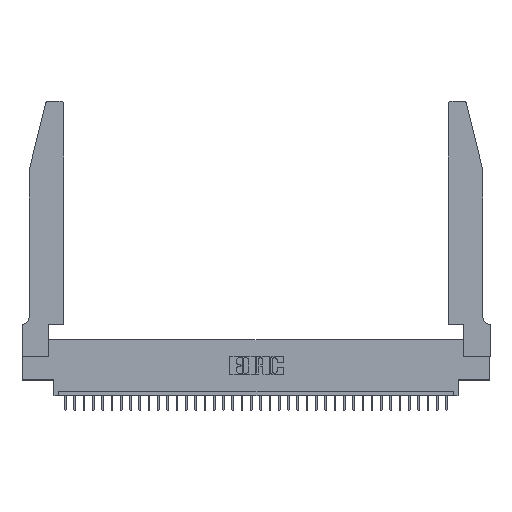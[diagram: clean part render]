
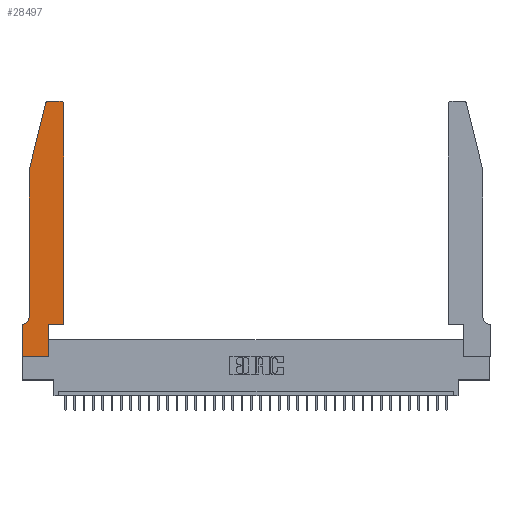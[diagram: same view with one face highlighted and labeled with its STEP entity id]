
A CAD part, top view. The second image highlights one B-rep face of the part: STEP entity #28497.
In plain terms, the highlighted planar face has unit normal (0, 0, 1).
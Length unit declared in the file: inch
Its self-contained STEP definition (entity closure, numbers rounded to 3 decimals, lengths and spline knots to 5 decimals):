
#23 = AXIS2_PLACEMENT_3D ( 'NONE', #22411, #19814, #30839 ) ;
#303 = DIRECTION ( 'NONE',  ( 0., 0., 1. ) ) ;
#573 = LINE ( 'NONE', #972, #12017 ) ;
#666 = EDGE_CURVE ( 'NONE', #1875, #23000, #20949, .T. ) ;
#972 = CARTESIAN_POINT ( 'NONE',  ( 0.2865, 0.35, 0.37 ) ) ;
#1875 = VERTEX_POINT ( 'NONE', #16837 ) ;
#1947 = PLANE ( 'NONE',  #32870 ) ;
#2014 = CARTESIAN_POINT ( 'NONE',  ( 0.4505, 0.35, 0.37 ) ) ;
#2196 = DIRECTION ( 'NONE',  ( 0., 1., 0. ) ) ;
#2394 = CARTESIAN_POINT ( 'NONE',  ( 0.4505, 2.72, 0.37 ) ) ;
#2555 = LINE ( 'NONE', #10203, #13099 ) ;
#2617 = CARTESIAN_POINT ( 'NONE',  ( 0.4205, 2.72, 0.37 ) ) ;
#2814 = EDGE_CURVE ( 'NONE', #3935, #32308, #13281, .T. ) ;
#2933 = EDGE_CURVE ( 'NONE', #7395, #24119, #9731, .T. ) ;
#3104 = CARTESIAN_POINT ( 'NONE',  ( 0., 0.35, 0.37 ) ) ;
#3274 = DIRECTION ( 'NONE',  ( 0., 0., 1. ) ) ;
#3289 = VERTEX_POINT ( 'NONE', #25113 ) ;
#3935 = VERTEX_POINT ( 'NONE', #27702 ) ;
#4242 = DIRECTION ( 'NONE',  ( -0.239, -0.971, 0. ) ) ;
#4882 = EDGE_CURVE ( 'NONE', #5404, #3289, #2555, .T. ) ;
#5018 = CARTESIAN_POINT ( 'NONE',  ( 0.0055, 0.35, 0.37 ) ) ;
#5260 = CIRCLE ( 'NONE', #9674, 0.03 ) ;
#5404 = VERTEX_POINT ( 'NONE', #26618 ) ;
#5456 = LINE ( 'NONE', #9632, #30645 ) ;
#6703 = VERTEX_POINT ( 'NONE', #7307 ) ;
#7047 = EDGE_CURVE ( 'NONE', #10008, #7395, #35138, .T. ) ;
#7307 = CARTESIAN_POINT ( 'NONE',  ( 0.2865, 0., 0.37 ) ) ;
#7395 = VERTEX_POINT ( 'NONE', #3104 ) ;
#7493 = EDGE_CURVE ( 'NONE', #24119, #6703, #25794, .T. ) ;
#7715 = VECTOR ( 'NONE', #22117, 39.37008 ) ;
#7849 = DIRECTION ( 'NONE',  ( 1., 0., 0. ) ) ;
#8033 = EDGE_CURVE ( 'NONE', #6703, #1875, #573, .T. ) ;
#9632 = CARTESIAN_POINT ( 'NONE',  ( 0.0755, 2., 0.37 ) ) ;
#9674 = AXIS2_PLACEMENT_3D ( 'NONE', #2617, #3274, #16997 ) ;
#9731 = LINE ( 'NONE', #20816, #12389 ) ;
#10008 = VERTEX_POINT ( 'NONE', #5018 ) ;
#10203 = CARTESIAN_POINT ( 'NONE',  ( 0.0755, 2., 0.37 ) ) ;
#10679 = CARTESIAN_POINT ( 'NONE',  ( 0., 0.35, 0.37 ) ) ;
#11181 = ORIENTED_EDGE ( 'NONE', *, *, #14940, .T. ) ;
#11901 = CARTESIAN_POINT ( 'NONE',  ( 0.2605, 2.75, 0.37 ) ) ;
#12017 = VECTOR ( 'NONE', #2196, 39.37008 ) ;
#12389 = VECTOR ( 'NONE', #12514, 39.37008 ) ;
#12490 = DIRECTION ( 'NONE',  ( -1., 0., 0. ) ) ;
#12514 = DIRECTION ( 'NONE',  ( 0., -1., 0. ) ) ;
#12538 = CARTESIAN_POINT ( 'NONE',  ( 0.284, 2.75, 0.37 ) ) ;
#13099 = VECTOR ( 'NONE', #26910, 39.37008 ) ;
#13281 = LINE ( 'NONE', #11901, #23899 ) ;
#13383 = DIRECTION ( 'NONE',  ( 1., 0., 0. ) ) ;
#13661 = VERTEX_POINT ( 'NONE', #25826 ) ;
#14126 = ORIENTED_EDGE ( 'NONE', *, *, #2814, .T. ) ;
#14582 = ORIENTED_EDGE ( 'NONE', *, *, #21919, .T. ) ;
#14605 = VECTOR ( 'NONE', #19224, 39.37008 ) ;
#14940 = EDGE_CURVE ( 'NONE', #23000, #23074, #34547, .T. ) ;
#15252 = ORIENTED_EDGE ( 'NONE', *, *, #666, .T. ) ;
#16066 = VECTOR ( 'NONE', #24854, 39.37008 ) ;
#16837 = CARTESIAN_POINT ( 'NONE',  ( 0.2865, 0.35, 0.37 ) ) ;
#16997 = DIRECTION ( 'NONE',  ( 1., 0., 0. ) ) ;
#17340 = ORIENTED_EDGE ( 'NONE', *, *, #8033, .T. ) ;
#17452 = CARTESIAN_POINT ( 'NONE',  ( 0.0755, 0.35, 0.37 ) ) ;
#18187 = ORIENTED_EDGE ( 'NONE', *, *, #30201, .T. ) ;
#19224 = DIRECTION ( 'NONE',  ( 0., 1., 0. ) ) ;
#19736 = EDGE_CURVE ( 'NONE', #32308, #13661, #23760, .T. ) ;
#19814 = DIRECTION ( 'NONE',  ( 0., 0., -1. ) ) ;
#20065 = VECTOR ( 'NONE', #12490, 39.37008 ) ;
#20454 = DIRECTION ( 'NONE',  ( -1., 0., 0. ) ) ;
#20494 = ORIENTED_EDGE ( 'NONE', *, *, #7493, .T. ) ;
#20816 = CARTESIAN_POINT ( 'NONE',  ( 0., 0., 0.37 ) ) ;
#20949 = LINE ( 'NONE', #26591, #7715 ) ;
#21100 = ORIENTED_EDGE ( 'NONE', *, *, #7047, .T. ) ;
#21771 = EDGE_LOOP ( 'NONE', ( #14126, #31903, #14582, #31843, #32867, #21100, #32551, #20494, #17340, #15252, #11181, #18187 ) ) ;
#21919 = EDGE_CURVE ( 'NONE', #13661, #5404, #5456, .T. ) ;
#22117 = DIRECTION ( 'NONE',  ( 1., 0., 0. ) ) ;
#22411 = CARTESIAN_POINT ( 'NONE',  ( 0.0055, 0.42, 0.37 ) ) ;
#23000 = VERTEX_POINT ( 'NONE', #2014 ) ;
#23049 = FACE_OUTER_BOUND ( 'NONE', #21771, .T. ) ;
#23074 = VERTEX_POINT ( 'NONE', #2394 ) ;
#23760 = CIRCLE ( 'NONE', #34315, 0.03 ) ;
#23899 = VECTOR ( 'NONE', #20454, 39.37008 ) ;
#24119 = VERTEX_POINT ( 'NONE', #29345 ) ;
#24854 = DIRECTION ( 'NONE',  ( 1., 0., 0. ) ) ;
#25113 = CARTESIAN_POINT ( 'NONE',  ( 0.0755, 0.42, 0.37 ) ) ;
#25794 = LINE ( 'NONE', #32726, #16066 ) ;
#25826 = CARTESIAN_POINT ( 'NONE',  ( 0.25487, 2.72718, 0.37 ) ) ;
#26591 = CARTESIAN_POINT ( 'NONE',  ( 0.4505, 0.35, 0.37 ) ) ;
#26618 = CARTESIAN_POINT ( 'NONE',  ( 0.0755, 2., 0.37 ) ) ;
#26910 = DIRECTION ( 'NONE',  ( 0., -1., 0. ) ) ;
#27702 = CARTESIAN_POINT ( 'NONE',  ( 0.4205, 2.75, 0.37 ) ) ;
#27990 = CARTESIAN_POINT ( 'NONE',  ( 0.4505, 0.35, 0.37 ) ) ;
#28497 = ADVANCED_FACE ( 'NONE', ( #23049 ), #1947, .T. ) ;
#29345 = CARTESIAN_POINT ( 'NONE',  ( 0., 0., 0.37 ) ) ;
#30201 = EDGE_CURVE ( 'NONE', #23074, #3935, #5260, .T. ) ;
#30316 = DIRECTION ( 'NONE',  ( 0., 0., 1. ) ) ;
#30645 = VECTOR ( 'NONE', #4242, 39.37008 ) ;
#30839 = DIRECTION ( 'NONE',  ( -1., 0., 0. ) ) ;
#31843 = ORIENTED_EDGE ( 'NONE', *, *, #4882, .T. ) ;
#31903 = ORIENTED_EDGE ( 'NONE', *, *, #19736, .T. ) ;
#32308 = VERTEX_POINT ( 'NONE', #12538 ) ;
#32551 = ORIENTED_EDGE ( 'NONE', *, *, #2933, .T. ) ;
#32726 = CARTESIAN_POINT ( 'NONE',  ( 0., 0., 0.37 ) ) ;
#32867 = ORIENTED_EDGE ( 'NONE', *, *, #35903, .T. ) ;
#32870 = AXIS2_PLACEMENT_3D ( 'NONE', #10679, #30316, #13383 ) ;
#33412 = CARTESIAN_POINT ( 'NONE',  ( 0.284, 2.72, 0.37 ) ) ;
#33848 = CIRCLE ( 'NONE', #23, 0.07 ) ;
#34315 = AXIS2_PLACEMENT_3D ( 'NONE', #33412, #303, #7849 ) ;
#34547 = LINE ( 'NONE', #27990, #14605 ) ;
#35138 = LINE ( 'NONE', #17452, #20065 ) ;
#35903 = EDGE_CURVE ( 'NONE', #3289, #10008, #33848, .T. ) ;
